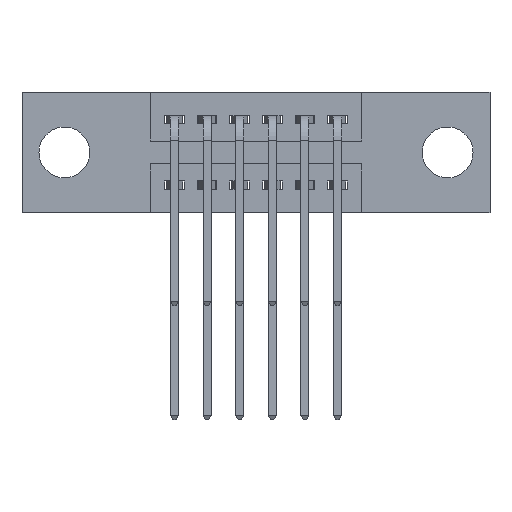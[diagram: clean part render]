
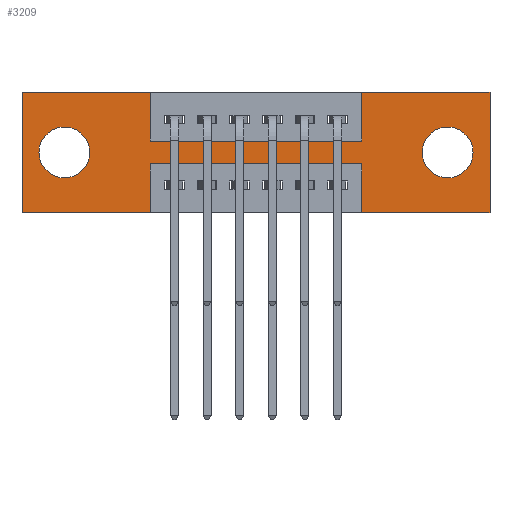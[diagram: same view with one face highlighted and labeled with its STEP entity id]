
A CAD part, front view. The second image highlights one B-rep face of the part: STEP entity #3209.
In plain terms, the highlighted planar face has unit normal (0, -1, 0).
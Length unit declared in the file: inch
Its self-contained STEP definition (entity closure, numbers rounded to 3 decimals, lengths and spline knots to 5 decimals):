
#27 = VERTEX_POINT ( 'NONE', #3549 ) ;
#119 = ORIENTED_EDGE ( 'NONE', *, *, #10202, .T. ) ;
#173 = CARTESIAN_POINT ( 'NONE',  ( 0.3925, 0., -0.37 ) ) ;
#199 = CARTESIAN_POINT ( 'NONE',  ( 1.435, 0., 0. ) ) ;
#254 = ORIENTED_EDGE ( 'NONE', *, *, #8920, .F. ) ;
#289 = DIRECTION ( 'NONE',  ( 0., 0., -1. ) ) ;
#320 = VERTEX_POINT ( 'NONE', #3361 ) ;
#418 = CARTESIAN_POINT ( 'NONE',  ( 0., 0., -0.37 ) ) ;
#492 = DIRECTION ( 'NONE',  ( 0., -1., 0. ) ) ;
#536 = ORIENTED_EDGE ( 'NONE', *, *, #5491, .F. ) ;
#581 = DIRECTION ( 'NONE',  ( 0., 0., -1. ) ) ;
#623 = DIRECTION ( 'NONE',  ( 0., 1., 0. ) ) ;
#780 = CARTESIAN_POINT ( 'NONE',  ( 1.0425, 0., -0.37 ) ) ;
#793 = VERTEX_POINT ( 'NONE', #4332 ) ;
#795 = VECTOR ( 'NONE', #8945, 39.37008 ) ;
#811 = LINE ( 'NONE', #3432, #3536 ) ;
#981 = VERTEX_POINT ( 'NONE', #3140 ) ;
#1288 = LINE ( 'NONE', #6330, #8205 ) ;
#1353 = VERTEX_POINT ( 'NONE', #199 ) ;
#1506 = CARTESIAN_POINT ( 'NONE',  ( 1.305, 0., -0.185 ) ) ;
#1761 = DIRECTION ( 'NONE',  ( 0., 0., 1. ) ) ;
#1787 = VERTEX_POINT ( 'NONE', #2676 ) ;
#1796 = CARTESIAN_POINT ( 'NONE',  ( 1.0425, 0., 0. ) ) ;
#1813 = AXIS2_PLACEMENT_3D ( 'NONE', #10960, #6287, #581 ) ;
#1975 = DIRECTION ( 'NONE',  ( 1., 0., 0. ) ) ;
#2075 = FACE_OUTER_BOUND ( 'NONE', #8355, .T. ) ;
#2224 = ORIENTED_EDGE ( 'NONE', *, *, #5955, .F. ) ;
#2562 = AXIS2_PLACEMENT_3D ( 'NONE', #6324, #623, #7149 ) ;
#2564 = DIRECTION ( 'NONE',  ( 0., 0., -1. ) ) ;
#2676 = CARTESIAN_POINT ( 'NONE',  ( 0.3925, 0., -0.22 ) ) ;
#2718 = CARTESIAN_POINT ( 'NONE',  ( 1.305, 0., -0.107 ) ) ;
#2888 = DIRECTION ( 'NONE',  ( 0., 0., 1. ) ) ;
#3111 = VERTEX_POINT ( 'NONE', #10988 ) ;
#3140 = CARTESIAN_POINT ( 'NONE',  ( 1.305, 0., -0.263 ) ) ;
#3177 = CIRCLE ( 'NONE', #8617, 0.078 ) ;
#3209 = ADVANCED_FACE ( 'NONE', ( #6750, #10623, #2075 ), #5755, .T. ) ;
#3305 = DIRECTION ( 'NONE',  ( 1., 0., 0. ) ) ;
#3361 = CARTESIAN_POINT ( 'NONE',  ( 1.0425, 0., 0. ) ) ;
#3387 = VECTOR ( 'NONE', #3305, 39.37008 ) ;
#3432 = CARTESIAN_POINT ( 'NONE',  ( 0., 0., 0. ) ) ;
#3536 = VECTOR ( 'NONE', #10077, 39.37008 ) ;
#3549 = CARTESIAN_POINT ( 'NONE',  ( 1.435, 0., -0.37 ) ) ;
#3674 = LINE ( 'NONE', #780, #7948 ) ;
#3785 = EDGE_LOOP ( 'NONE', ( #5657, #119 ) ) ;
#3791 = VECTOR ( 'NONE', #7364, 39.37008 ) ;
#4000 = LINE ( 'NONE', #7225, #10461 ) ;
#4056 = CARTESIAN_POINT ( 'NONE',  ( 0.3925, 0., -0.15 ) ) ;
#4178 = VERTEX_POINT ( 'NONE', #173 ) ;
#4181 = CARTESIAN_POINT ( 'NONE',  ( 0., 0., -0.37 ) ) ;
#4212 = CARTESIAN_POINT ( 'NONE',  ( 0.13, 0., -0.185 ) ) ;
#4332 = CARTESIAN_POINT ( 'NONE',  ( 1.0425, 0., -0.22 ) ) ;
#4336 = CARTESIAN_POINT ( 'NONE',  ( 0.3925, 0., 0. ) ) ;
#4358 = VERTEX_POINT ( 'NONE', #9657 ) ;
#4581 = EDGE_CURVE ( 'NONE', #320, #1353, #10037, .T. ) ;
#4631 = CIRCLE ( 'NONE', #2562, 0.078 ) ;
#4852 = VERTEX_POINT ( 'NONE', #2718 ) ;
#4906 = ORIENTED_EDGE ( 'NONE', *, *, #7142, .F. ) ;
#4915 = VERTEX_POINT ( 'NONE', #5613 ) ;
#5109 = DIRECTION ( 'NONE',  ( 0., 0., 1. ) ) ;
#5196 = ORIENTED_EDGE ( 'NONE', *, *, #7293, .F. ) ;
#5282 = LINE ( 'NONE', #1796, #9295 ) ;
#5325 = ORIENTED_EDGE ( 'NONE', *, *, #6969, .T. ) ;
#5447 = CARTESIAN_POINT ( 'NONE',  ( 0., 0., 0. ) ) ;
#5491 = EDGE_CURVE ( 'NONE', #8304, #11192, #811, .T. ) ;
#5538 = ORIENTED_EDGE ( 'NONE', *, *, #7525, .F. ) ;
#5613 = CARTESIAN_POINT ( 'NONE',  ( 0.13, 0., -0.107 ) ) ;
#5653 = AXIS2_PLACEMENT_3D ( 'NONE', #1506, #7874, #2564 ) ;
#5657 = ORIENTED_EDGE ( 'NONE', *, *, #6924, .T. ) ;
#5692 = EDGE_CURVE ( 'NONE', #1353, #27, #1288, .T. ) ;
#5755 = PLANE ( 'NONE',  #10827 ) ;
#5955 = EDGE_CURVE ( 'NONE', #27, #3111, #8084, .T. ) ;
#6056 = VECTOR ( 'NONE', #11049, 39.37008 ) ;
#6186 = VECTOR ( 'NONE', #1975, 39.37008 ) ;
#6287 = DIRECTION ( 'NONE',  ( 0., 1., 0. ) ) ;
#6315 = ORIENTED_EDGE ( 'NONE', *, *, #7028, .F. ) ;
#6324 = CARTESIAN_POINT ( 'NONE',  ( 0.13, 0., -0.185 ) ) ;
#6330 = CARTESIAN_POINT ( 'NONE',  ( 1.435, 0., 0. ) ) ;
#6389 = EDGE_CURVE ( 'NONE', #4178, #8304, #10823, .T. ) ;
#6520 = EDGE_CURVE ( 'NONE', #4358, #4915, #3177, .T. ) ;
#6549 = LINE ( 'NONE', #4336, #10450 ) ;
#6750 = FACE_BOUND ( 'NONE', #3785, .T. ) ;
#6924 = EDGE_CURVE ( 'NONE', #4852, #981, #9176, .T. ) ;
#6955 = VECTOR ( 'NONE', #9313, 39.37008 ) ;
#6969 = EDGE_CURVE ( 'NONE', #4915, #4358, #4631, .T. ) ;
#6985 = VERTEX_POINT ( 'NONE', #10983 ) ;
#7028 = EDGE_CURVE ( 'NONE', #1787, #4178, #4000, .T. ) ;
#7030 = CIRCLE ( 'NONE', #5653, 0.078 ) ;
#7040 = EDGE_CURVE ( 'NONE', #793, #1787, #8443, .T. ) ;
#7088 = ORIENTED_EDGE ( 'NONE', *, *, #4581, .F. ) ;
#7094 = EDGE_CURVE ( 'NONE', #3111, #793, #3674, .T. ) ;
#7142 = EDGE_CURVE ( 'NONE', #6985, #320, #5282, .T. ) ;
#7149 = DIRECTION ( 'NONE',  ( 0., 0., 1. ) ) ;
#7225 = CARTESIAN_POINT ( 'NONE',  ( 0.3925, 0., -0.37 ) ) ;
#7293 = EDGE_CURVE ( 'NONE', #9634, #6985, #8314, .T. ) ;
#7364 = DIRECTION ( 'NONE',  ( 1., 0., 0. ) ) ;
#7432 = DIRECTION ( 'NONE',  ( 0., 0., -1. ) ) ;
#7525 = EDGE_CURVE ( 'NONE', #7852, #9634, #6549, .T. ) ;
#7706 = ORIENTED_EDGE ( 'NONE', *, *, #6389, .F. ) ;
#7761 = EDGE_LOOP ( 'NONE', ( #5325, #8449 ) ) ;
#7852 = VERTEX_POINT ( 'NONE', #8755 ) ;
#7874 = DIRECTION ( 'NONE',  ( 0., 1., 0. ) ) ;
#7948 = VECTOR ( 'NONE', #1761, 39.37008 ) ;
#8019 = DIRECTION ( 'NONE',  ( 0., 0., -1. ) ) ;
#8084 = LINE ( 'NONE', #8153, #795 ) ;
#8153 = CARTESIAN_POINT ( 'NONE',  ( 0., 0., -0.37 ) ) ;
#8205 = VECTOR ( 'NONE', #9478, 39.37008 ) ;
#8304 = VERTEX_POINT ( 'NONE', #4181 ) ;
#8314 = LINE ( 'NONE', #4056, #6186 ) ;
#8355 = EDGE_LOOP ( 'NONE', ( #6315, #8691, #10471, #2224, #10727, #7088, #4906, #5196, #5538, #254, #536, #7706 ) ) ;
#8443 = LINE ( 'NONE', #9538, #6056 ) ;
#8449 = ORIENTED_EDGE ( 'NONE', *, *, #6520, .T. ) ;
#8450 = CARTESIAN_POINT ( 'NONE',  ( 0., 0., 0. ) ) ;
#8523 = LINE ( 'NONE', #11199, #3791 ) ;
#8617 = AXIS2_PLACEMENT_3D ( 'NONE', #4212, #9877, #5109 ) ;
#8691 = ORIENTED_EDGE ( 'NONE', *, *, #7040, .F. ) ;
#8755 = CARTESIAN_POINT ( 'NONE',  ( 0.3925, 0., 0. ) ) ;
#8920 = EDGE_CURVE ( 'NONE', #11192, #7852, #8523, .T. ) ;
#8945 = DIRECTION ( 'NONE',  ( -1., 0., 0. ) ) ;
#9136 = CARTESIAN_POINT ( 'NONE',  ( 0., 0., -0.37 ) ) ;
#9176 = CIRCLE ( 'NONE', #1813, 0.078 ) ;
#9295 = VECTOR ( 'NONE', #2888, 39.37008 ) ;
#9313 = DIRECTION ( 'NONE',  ( -1., 0., 0. ) ) ;
#9478 = DIRECTION ( 'NONE',  ( 0., 0., -1. ) ) ;
#9538 = CARTESIAN_POINT ( 'NONE',  ( 0.3925, 0., -0.22 ) ) ;
#9634 = VERTEX_POINT ( 'NONE', #10324 ) ;
#9657 = CARTESIAN_POINT ( 'NONE',  ( 0.13, 0., -0.263 ) ) ;
#9877 = DIRECTION ( 'NONE',  ( 0., 1., 0. ) ) ;
#10037 = LINE ( 'NONE', #8450, #3387 ) ;
#10077 = DIRECTION ( 'NONE',  ( 0., 0., 1. ) ) ;
#10202 = EDGE_CURVE ( 'NONE', #981, #4852, #7030, .T. ) ;
#10324 = CARTESIAN_POINT ( 'NONE',  ( 0.3925, 0., -0.15 ) ) ;
#10450 = VECTOR ( 'NONE', #289, 39.37008 ) ;
#10461 = VECTOR ( 'NONE', #8019, 39.37008 ) ;
#10471 = ORIENTED_EDGE ( 'NONE', *, *, #7094, .F. ) ;
#10623 = FACE_BOUND ( 'NONE', #7761, .T. ) ;
#10727 = ORIENTED_EDGE ( 'NONE', *, *, #5692, .F. ) ;
#10823 = LINE ( 'NONE', #418, #6955 ) ;
#10827 = AXIS2_PLACEMENT_3D ( 'NONE', #9136, #492, #7432 ) ;
#10960 = CARTESIAN_POINT ( 'NONE',  ( 1.305, 0., -0.185 ) ) ;
#10983 = CARTESIAN_POINT ( 'NONE',  ( 1.0425, 0., -0.15 ) ) ;
#10988 = CARTESIAN_POINT ( 'NONE',  ( 1.0425, 0., -0.37 ) ) ;
#11049 = DIRECTION ( 'NONE',  ( -1., 0., 0. ) ) ;
#11192 = VERTEX_POINT ( 'NONE', #5447 ) ;
#11199 = CARTESIAN_POINT ( 'NONE',  ( 0., 0., 0. ) ) ;
